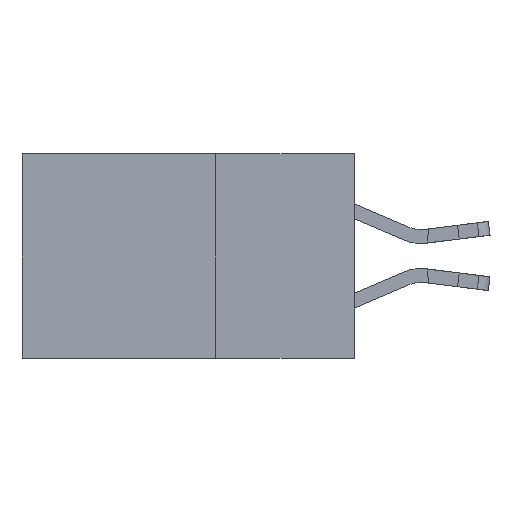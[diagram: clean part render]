
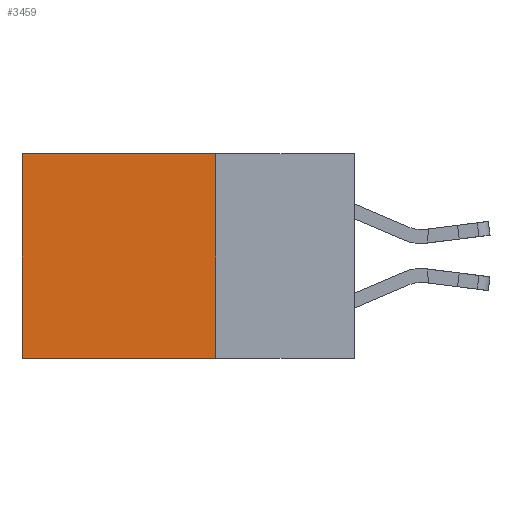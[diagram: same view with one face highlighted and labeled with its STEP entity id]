
A CAD part, left-side view. The second image highlights one B-rep face of the part: STEP entity #3459.
In plain terms, the highlighted planar face has unit normal (-1, 0, 0).
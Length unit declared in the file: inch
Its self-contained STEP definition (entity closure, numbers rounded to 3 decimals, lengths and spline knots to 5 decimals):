
#340 = VECTOR ( 'NONE', #3800, 39.37008 ) ;
#590 = DIRECTION ( 'NONE',  ( 1., 0., 0. ) ) ;
#935 = LINE ( 'NONE', #4877, #3130 ) ;
#1514 = ORIENTED_EDGE ( 'NONE', *, *, #9089, .T. ) ;
#1555 = ORIENTED_EDGE ( 'NONE', *, *, #2831, .F. ) ;
#1932 = CARTESIAN_POINT ( 'NONE',  ( 0.2615, 0.25, 0. ) ) ;
#2290 = VERTEX_POINT ( 'NONE', #6874 ) ;
#2831 = EDGE_CURVE ( 'NONE', #2290, #8704, #10029, .T. ) ;
#2834 = FACE_OUTER_BOUND ( 'NONE', #8107, .T. ) ;
#2871 = DIRECTION ( 'NONE',  ( 0., 0., -1. ) ) ;
#2995 = VECTOR ( 'NONE', #8184, 39.37008 ) ;
#3008 = EDGE_CURVE ( 'NONE', #3275, #8704, #935, .T. ) ;
#3090 = CARTESIAN_POINT ( 'NONE',  ( 0.2615, 0.25, 0. ) ) ;
#3114 = CARTESIAN_POINT ( 'NONE',  ( 0.2615, 0.25, -0.37 ) ) ;
#3130 = VECTOR ( 'NONE', #4837, 39.37008 ) ;
#3275 = VERTEX_POINT ( 'NONE', #10734 ) ;
#3284 = EDGE_CURVE ( 'NONE', #10413, #2290, #5156, .T. ) ;
#3295 = PLANE ( 'NONE',  #7427 ) ;
#3459 = ADVANCED_FACE ( 'NONE', ( #2834 ), #3295, .F. ) ;
#3800 = DIRECTION ( 'NONE',  ( 0., 1., 0. ) ) ;
#4837 = DIRECTION ( 'NONE',  ( 0., 0., -1. ) ) ;
#4877 = CARTESIAN_POINT ( 'NONE',  ( 0.2615, 0.6, -0.37 ) ) ;
#5156 = LINE ( 'NONE', #10995, #11876 ) ;
#6874 = CARTESIAN_POINT ( 'NONE',  ( 0.2615, 0.25, -0.37 ) ) ;
#7427 = AXIS2_PLACEMENT_3D ( 'NONE', #3114, #590, #2871 ) ;
#7973 = ORIENTED_EDGE ( 'NONE', *, *, #3008, .T. ) ;
#8107 = EDGE_LOOP ( 'NONE', ( #7973, #1555, #10338, #1514 ) ) ;
#8184 = DIRECTION ( 'NONE',  ( 0., 1., 0. ) ) ;
#8276 = CARTESIAN_POINT ( 'NONE',  ( 0.2615, 0.25, -0.37 ) ) ;
#8704 = VERTEX_POINT ( 'NONE', #11444 ) ;
#9089 = EDGE_CURVE ( 'NONE', #10413, #3275, #10158, .T. ) ;
#10029 = LINE ( 'NONE', #8276, #2995 ) ;
#10086 = DIRECTION ( 'NONE',  ( 0., 0., -1. ) ) ;
#10158 = LINE ( 'NONE', #1932, #340 ) ;
#10338 = ORIENTED_EDGE ( 'NONE', *, *, #3284, .F. ) ;
#10413 = VERTEX_POINT ( 'NONE', #3090 ) ;
#10734 = CARTESIAN_POINT ( 'NONE',  ( 0.2615, 0.6, 0. ) ) ;
#10995 = CARTESIAN_POINT ( 'NONE',  ( 0.2615, 0.25, -0.37 ) ) ;
#11444 = CARTESIAN_POINT ( 'NONE',  ( 0.2615, 0.6, -0.37 ) ) ;
#11876 = VECTOR ( 'NONE', #10086, 39.37008 ) ;
